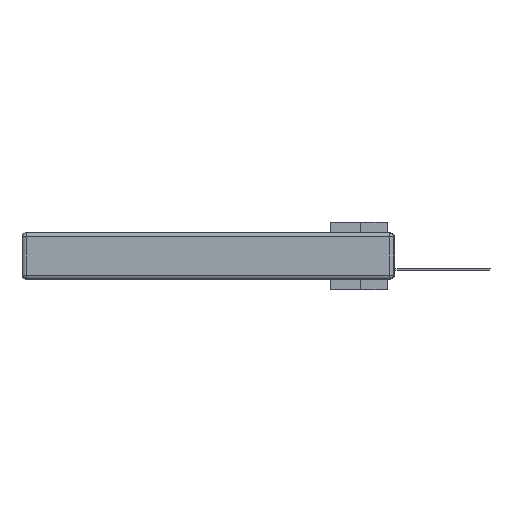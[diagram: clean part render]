
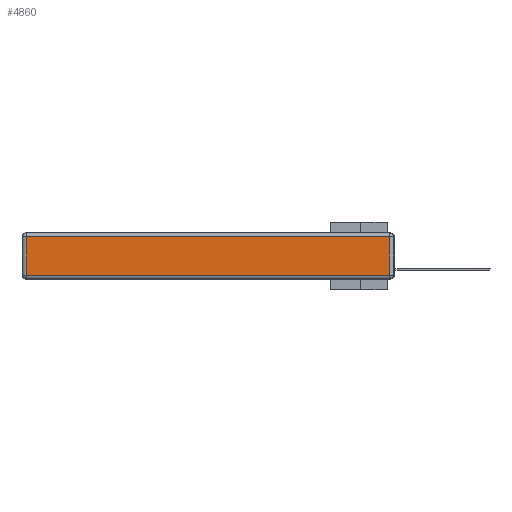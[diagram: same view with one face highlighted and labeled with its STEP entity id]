
A CAD part, left-side view. The second image highlights one B-rep face of the part: STEP entity #4860.
In plain terms, the highlighted planar face has unit normal (-1, 0, 0).
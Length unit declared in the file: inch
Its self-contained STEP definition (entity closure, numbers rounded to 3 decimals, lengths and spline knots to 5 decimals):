
#216 = ORIENTED_EDGE ( 'NONE', *, *, #34705, .T. ) ;
#662 = VECTOR ( 'NONE', #21797, 39.37008 ) ;
#1544 = ORIENTED_EDGE ( 'NONE', *, *, #23502, .T. ) ;
#2485 = VERTEX_POINT ( 'NONE', #35920 ) ;
#4312 = VERTEX_POINT ( 'NONE', #28469 ) ;
#4860 = ADVANCED_FACE ( 'NONE', ( #28826 ), #22621, .T. ) ;
#4970 = CARTESIAN_POINT ( 'NONE',  ( 0., 0.03, -0.343 ) ) ;
#5051 = CARTESIAN_POINT ( 'NONE',  ( 0., 0., -0.343 ) ) ;
#8236 = DIRECTION ( 'NONE',  ( 0., 0., 1. ) ) ;
#9317 = EDGE_CURVE ( 'NONE', #34272, #4312, #31276, .T. ) ;
#10182 = VERTEX_POINT ( 'NONE', #11861 ) ;
#11371 = CARTESIAN_POINT ( 'NONE',  ( 0., 2.72, -0.343 ) ) ;
#11861 = CARTESIAN_POINT ( 'NONE',  ( 0., 0.03, -0.313 ) ) ;
#13764 = DIRECTION ( 'NONE',  ( 0., 0., -1. ) ) ;
#15269 = EDGE_LOOP ( 'NONE', ( #216, #28376, #1544, #33215 ) ) ;
#16182 = VECTOR ( 'NONE', #13764, 39.37008 ) ;
#18729 = VECTOR ( 'NONE', #26792, 39.37008 ) ;
#20700 = EDGE_CURVE ( 'NONE', #10182, #2485, #35873, .T. ) ;
#20868 = AXIS2_PLACEMENT_3D ( 'NONE', #5051, #25597, #8236 ) ;
#21797 = DIRECTION ( 'NONE',  ( 0., 1., 0. ) ) ;
#22621 = PLANE ( 'NONE',  #20868 ) ;
#23502 = EDGE_CURVE ( 'NONE', #2485, #34272, #31549, .T. ) ;
#25163 = CARTESIAN_POINT ( 'NONE',  ( 0., 2.72, -0.03 ) ) ;
#25530 = DIRECTION ( 'NONE',  ( 0., 0., 1. ) ) ;
#25597 = DIRECTION ( 'NONE',  ( -1., 0., 0. ) ) ;
#26792 = DIRECTION ( 'NONE',  ( 0., -1., 0. ) ) ;
#28160 = VECTOR ( 'NONE', #25530, 39.37008 ) ;
#28376 = ORIENTED_EDGE ( 'NONE', *, *, #20700, .T. ) ;
#28469 = CARTESIAN_POINT ( 'NONE',  ( 0., 2.72, -0.313 ) ) ;
#28826 = FACE_OUTER_BOUND ( 'NONE', #15269, .T. ) ;
#31276 = LINE ( 'NONE', #11371, #16182 ) ;
#31549 = LINE ( 'NONE', #33372, #662 ) ;
#32094 = LINE ( 'NONE', #32451, #18729 ) ;
#32451 = CARTESIAN_POINT ( 'NONE',  ( 0., 0., -0.313 ) ) ;
#33215 = ORIENTED_EDGE ( 'NONE', *, *, #9317, .T. ) ;
#33372 = CARTESIAN_POINT ( 'NONE',  ( 0., 2.75, -0.03 ) ) ;
#34272 = VERTEX_POINT ( 'NONE', #25163 ) ;
#34705 = EDGE_CURVE ( 'NONE', #4312, #10182, #32094, .T. ) ;
#35873 = LINE ( 'NONE', #4970, #28160 ) ;
#35920 = CARTESIAN_POINT ( 'NONE',  ( 0., 0.03, -0.03 ) ) ;
